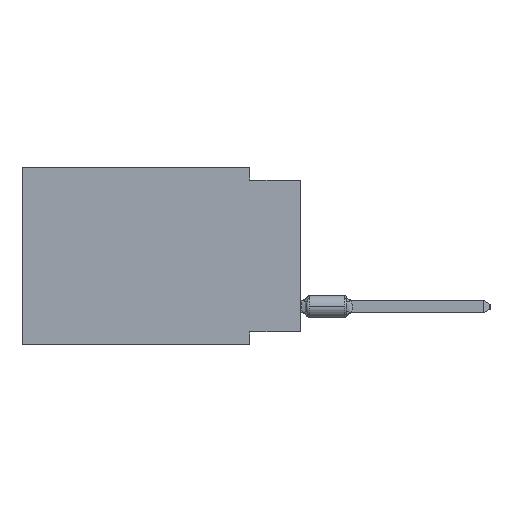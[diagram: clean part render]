
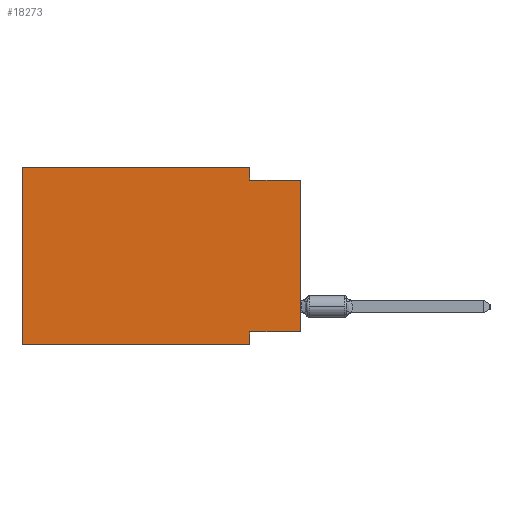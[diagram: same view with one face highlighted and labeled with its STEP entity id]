
A CAD part, left-side view. The second image highlights one B-rep face of the part: STEP entity #18273.
In plain terms, the highlighted planar face has unit normal (-1, 0, 0).
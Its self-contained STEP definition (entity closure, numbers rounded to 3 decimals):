
#587 = CARTESIAN_POINT ( 'NONE',  ( 0., 0., -8.255 ) ) ;
#1606 = CARTESIAN_POINT ( 'NONE',  ( 0., 13.97, 0. ) ) ;
#2788 = LINE ( 'NONE', #55344, #5415 ) ;
#4543 = DIRECTION ( 'NONE',  ( 0., 0., 1. ) ) ;
#4584 = VECTOR ( 'NONE', #4543, 1000. ) ;
#5415 = VECTOR ( 'NONE', #36229, 1000. ) ;
#6050 = CARTESIAN_POINT ( 'NONE',  ( 0., 2.54, 0. ) ) ;
#6104 = DIRECTION ( 'NONE',  ( 0., -1., 0. ) ) ;
#6583 = ORIENTED_EDGE ( 'NONE', *, *, #54012, .F. ) ;
#7700 = VERTEX_POINT ( 'NONE', #16119 ) ;
#9000 = LINE ( 'NONE', #22698, #4584 ) ;
#10148 = CARTESIAN_POINT ( 'NONE',  ( 0., 2.54, -8.255 ) ) ;
#10275 = DIRECTION ( 'NONE',  ( 1., 0., 0. ) ) ;
#10344 = VERTEX_POINT ( 'NONE', #50233 ) ;
#10392 = VERTEX_POINT ( 'NONE', #22552 ) ;
#13022 = LINE ( 'NONE', #41627, #32746 ) ;
#15043 = PLANE ( 'NONE',  #15078 ) ;
#15078 = AXIS2_PLACEMENT_3D ( 'NONE', #53831, #10275, #29682 ) ;
#15203 = EDGE_CURVE ( 'NONE', #26202, #7700, #57148, .T. ) ;
#16119 = CARTESIAN_POINT ( 'NONE',  ( 0., 2.54, -8.89 ) ) ;
#16306 = LINE ( 'NONE', #49672, #22671 ) ;
#18273 = ADVANCED_FACE ( 'NONE', ( #44573 ), #15043, .F. ) ;
#19536 = LINE ( 'NONE', #38585, #53298 ) ;
#22454 = CARTESIAN_POINT ( 'NONE',  ( 0., 13.97, -8.89 ) ) ;
#22552 = CARTESIAN_POINT ( 'NONE',  ( 0., 2.54, -0.635 ) ) ;
#22671 = VECTOR ( 'NONE', #6104, 1000. ) ;
#22698 = CARTESIAN_POINT ( 'NONE',  ( 0., 13.97, 0. ) ) ;
#23117 = EDGE_CURVE ( 'NONE', #53727, #58465, #13022, .T. ) ;
#24292 = EDGE_CURVE ( 'NONE', #10392, #58465, #16306, .T. ) ;
#24560 = LINE ( 'NONE', #6050, #46603 ) ;
#24893 = CARTESIAN_POINT ( 'NONE',  ( 0., 13.97, -8.89 ) ) ;
#26146 = EDGE_CURVE ( 'NONE', #26202, #40037, #9000, .T. ) ;
#26202 = VERTEX_POINT ( 'NONE', #24893 ) ;
#27853 = ORIENTED_EDGE ( 'NONE', *, *, #41346, .F. ) ;
#29639 = CARTESIAN_POINT ( 'NONE',  ( 0., 0., -0.635 ) ) ;
#29682 = DIRECTION ( 'NONE',  ( 0., 0., -1. ) ) ;
#30445 = ORIENTED_EDGE ( 'NONE', *, *, #15203, .T. ) ;
#32375 = LINE ( 'NONE', #42864, #62031 ) ;
#32746 = VECTOR ( 'NONE', #61075, 1000. ) ;
#33475 = ORIENTED_EDGE ( 'NONE', *, *, #42408, .F. ) ;
#33904 = ORIENTED_EDGE ( 'NONE', *, *, #24292, .F. ) ;
#36229 = DIRECTION ( 'NONE',  ( 0., 0., -1. ) ) ;
#36574 = ORIENTED_EDGE ( 'NONE', *, *, #26146, .F. ) ;
#37413 = ORIENTED_EDGE ( 'NONE', *, *, #23117, .T. ) ;
#37847 = EDGE_LOOP ( 'NONE', ( #37413, #33904, #61999, #33475, #36574, #30445, #27853, #6583 ) ) ;
#38585 = CARTESIAN_POINT ( 'NONE',  ( 0., 13.97, 0. ) ) ;
#39141 = VERTEX_POINT ( 'NONE', #10148 ) ;
#40037 = VERTEX_POINT ( 'NONE', #1606 ) ;
#41346 = EDGE_CURVE ( 'NONE', #39141, #7700, #2788, .T. ) ;
#41627 = CARTESIAN_POINT ( 'NONE',  ( 0., 0., 0. ) ) ;
#42408 = EDGE_CURVE ( 'NONE', #40037, #10344, #19536, .T. ) ;
#42864 = CARTESIAN_POINT ( 'NONE',  ( 0., 0., -8.255 ) ) ;
#44573 = FACE_OUTER_BOUND ( 'NONE', #37847, .T. ) ;
#46603 = VECTOR ( 'NONE', #59522, 1000. ) ;
#49672 = CARTESIAN_POINT ( 'NONE',  ( 0., 0., -0.635 ) ) ;
#50233 = CARTESIAN_POINT ( 'NONE',  ( 0., 2.54, 0. ) ) ;
#53298 = VECTOR ( 'NONE', #58022, 1000. ) ;
#53727 = VERTEX_POINT ( 'NONE', #587 ) ;
#53831 = CARTESIAN_POINT ( 'NONE',  ( 0., 13.97, 0. ) ) ;
#54012 = EDGE_CURVE ( 'NONE', #53727, #39141, #32375, .T. ) ;
#55344 = CARTESIAN_POINT ( 'NONE',  ( 0., 2.54, -8.89 ) ) ;
#56807 = DIRECTION ( 'NONE',  ( 0., -1., 0. ) ) ;
#57148 = LINE ( 'NONE', #22454, #57236 ) ;
#57236 = VECTOR ( 'NONE', #56807, 1000. ) ;
#58022 = DIRECTION ( 'NONE',  ( 0., -1., 0. ) ) ;
#58465 = VERTEX_POINT ( 'NONE', #29639 ) ;
#58490 = EDGE_CURVE ( 'NONE', #10344, #10392, #24560, .T. ) ;
#59522 = DIRECTION ( 'NONE',  ( 0., 0., -1. ) ) ;
#61075 = DIRECTION ( 'NONE',  ( 0., 0., 1. ) ) ;
#61999 = ORIENTED_EDGE ( 'NONE', *, *, #58490, .F. ) ;
#62031 = VECTOR ( 'NONE', #62312, 1000. ) ;
#62312 = DIRECTION ( 'NONE',  ( 0., 1., 0. ) ) ;
